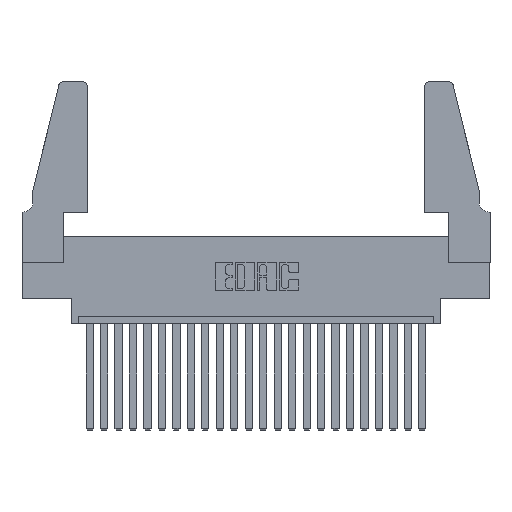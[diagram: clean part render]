
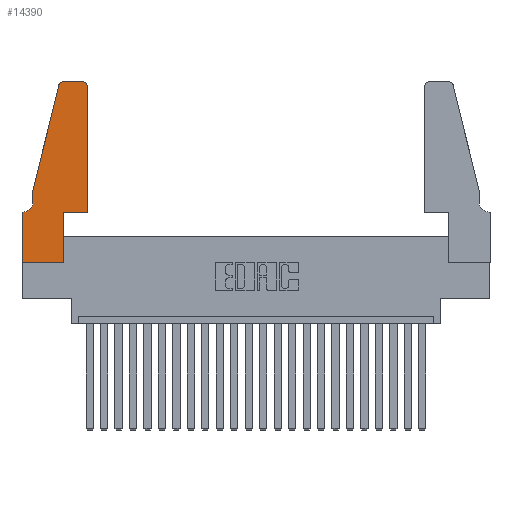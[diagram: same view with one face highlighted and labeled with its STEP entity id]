
A CAD part, top view. The second image highlights one B-rep face of the part: STEP entity #14390.
In plain terms, the highlighted planar face has unit normal (0, 0, 1).
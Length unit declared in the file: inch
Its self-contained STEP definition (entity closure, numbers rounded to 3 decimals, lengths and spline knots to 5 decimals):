
#561 = DIRECTION ( 'NONE',  ( 0., -1., 0. ) ) ;
#1116 = ORIENTED_EDGE ( 'NONE', *, *, #19696, .T. ) ;
#1305 = CARTESIAN_POINT ( 'NONE',  ( 0.4205, 1.22, 0.37 ) ) ;
#1450 = LINE ( 'NONE', #10555, #19457 ) ;
#1609 = VERTEX_POINT ( 'NONE', #7584 ) ;
#1665 = DIRECTION ( 'NONE',  ( 0., 0., 1. ) ) ;
#1676 = VERTEX_POINT ( 'NONE', #2249 ) ;
#1792 = EDGE_CURVE ( 'NONE', #5726, #1676, #8718, .T. ) ;
#1910 = DIRECTION ( 'NONE',  ( -0.239, -0.971, 0. ) ) ;
#2001 = CARTESIAN_POINT ( 'NONE',  ( 0., 0.35, 0.37 ) ) ;
#2024 = EDGE_LOOP ( 'NONE', ( #13230, #1116, #7763, #14770, #7213, #21778, #20930, #15979, #6445, #11899, #16811, #20175 ) ) ;
#2026 = EDGE_CURVE ( 'NONE', #1676, #17543, #18436, .T. ) ;
#2249 = CARTESIAN_POINT ( 'NONE',  ( 0., 0., 0.37 ) ) ;
#2500 = VECTOR ( 'NONE', #14699, 39.37008 ) ;
#3190 = VECTOR ( 'NONE', #20352, 39.37008 ) ;
#3226 = CARTESIAN_POINT ( 'NONE',  ( 0.284, 1.22, 0.37 ) ) ;
#3441 = CARTESIAN_POINT ( 'NONE',  ( 0., 0.35, 0.37 ) ) ;
#3914 = CIRCLE ( 'NONE', #15647, 0.03 ) ;
#4286 = EDGE_CURVE ( 'NONE', #7462, #20144, #18854, .T. ) ;
#4609 = EDGE_CURVE ( 'NONE', #1609, #6643, #7204, .T. ) ;
#4746 = VECTOR ( 'NONE', #1910, 39.37008 ) ;
#5726 = VERTEX_POINT ( 'NONE', #2001 ) ;
#6085 = DIRECTION ( 'NONE',  ( -1., 0., 0. ) ) ;
#6445 = ORIENTED_EDGE ( 'NONE', *, *, #7154, .T. ) ;
#6475 = CARTESIAN_POINT ( 'NONE',  ( 0., 0., 0.37 ) ) ;
#6643 = VERTEX_POINT ( 'NONE', #20934 ) ;
#7027 = DIRECTION ( 'NONE',  ( 0., 0., 1. ) ) ;
#7035 = LINE ( 'NONE', #17902, #19211 ) ;
#7154 = EDGE_CURVE ( 'NONE', #17543, #19338, #8972, .T. ) ;
#7204 = LINE ( 'NONE', #16432, #2500 ) ;
#7213 = ORIENTED_EDGE ( 'NONE', *, *, #11035, .T. ) ;
#7355 = CARTESIAN_POINT ( 'NONE',  ( 0.0755, 0.35, 0.37 ) ) ;
#7462 = VERTEX_POINT ( 'NONE', #18083 ) ;
#7584 = CARTESIAN_POINT ( 'NONE',  ( 0.4505, 0.35, 0.37 ) ) ;
#7623 = CARTESIAN_POINT ( 'NONE',  ( 0.0055, 0.35, 0.37 ) ) ;
#7763 = ORIENTED_EDGE ( 'NONE', *, *, #4286, .T. ) ;
#7776 = VERTEX_POINT ( 'NONE', #7623 ) ;
#8060 = DIRECTION ( 'NONE',  ( 1., 0., 0. ) ) ;
#8718 = LINE ( 'NONE', #9415, #11935 ) ;
#8972 = LINE ( 'NONE', #21272, #21488 ) ;
#9415 = CARTESIAN_POINT ( 'NONE',  ( 0., 0., 0.37 ) ) ;
#9448 = CARTESIAN_POINT ( 'NONE',  ( 0.2605, 1.25, 0.37 ) ) ;
#9596 = CIRCLE ( 'NONE', #12910, 0.03 ) ;
#9640 = VECTOR ( 'NONE', #15904, 39.37008 ) ;
#9907 = AXIS2_PLACEMENT_3D ( 'NONE', #22009, #16769, #18303 ) ;
#9958 = CARTESIAN_POINT ( 'NONE',  ( 0.2865, 0.35, 0.37 ) ) ;
#10555 = CARTESIAN_POINT ( 'NONE',  ( 0.0755, 0.5, 0.37 ) ) ;
#10727 = DIRECTION ( 'NONE',  ( 1., 0., 0. ) ) ;
#10754 = EDGE_CURVE ( 'NONE', #20144, #18884, #1450, .T. ) ;
#11035 = EDGE_CURVE ( 'NONE', #18884, #7776, #11817, .T. ) ;
#11658 = EDGE_CURVE ( 'NONE', #14169, #16993, #18050, .T. ) ;
#11817 = CIRCLE ( 'NONE', #9907, 0.07 ) ;
#11824 = DIRECTION ( 'NONE',  ( 1., 0., 0. ) ) ;
#11899 = ORIENTED_EDGE ( 'NONE', *, *, #15185, .T. ) ;
#11916 = DIRECTION ( 'NONE',  ( 1., 0., 0. ) ) ;
#11935 = VECTOR ( 'NONE', #18176, 39.37008 ) ;
#12910 = AXIS2_PLACEMENT_3D ( 'NONE', #3226, #1665, #11824 ) ;
#12967 = PLANE ( 'NONE',  #21171 ) ;
#13146 = VECTOR ( 'NONE', #6085, 39.37008 ) ;
#13230 = ORIENTED_EDGE ( 'NONE', *, *, #11658, .T. ) ;
#14169 = VERTEX_POINT ( 'NONE', #16796 ) ;
#14390 = ADVANCED_FACE ( 'NONE', ( #22054 ), #12967, .T. ) ;
#14699 = DIRECTION ( 'NONE',  ( 0., 1., 0. ) ) ;
#14770 = ORIENTED_EDGE ( 'NONE', *, *, #10754, .T. ) ;
#15185 = EDGE_CURVE ( 'NONE', #19338, #1609, #7035, .T. ) ;
#15647 = AXIS2_PLACEMENT_3D ( 'NONE', #1305, #7027, #11916 ) ;
#15904 = DIRECTION ( 'NONE',  ( -1., 0., 0. ) ) ;
#15979 = ORIENTED_EDGE ( 'NONE', *, *, #2026, .T. ) ;
#16432 = CARTESIAN_POINT ( 'NONE',  ( 0.4505, 0.35, 0.37 ) ) ;
#16769 = DIRECTION ( 'NONE',  ( 0., 0., -1. ) ) ;
#16796 = CARTESIAN_POINT ( 'NONE',  ( 0.4205, 1.25, 0.37 ) ) ;
#16811 = ORIENTED_EDGE ( 'NONE', *, *, #4609, .T. ) ;
#16993 = VERTEX_POINT ( 'NONE', #18685 ) ;
#17012 = EDGE_CURVE ( 'NONE', #6643, #14169, #3914, .T. ) ;
#17543 = VERTEX_POINT ( 'NONE', #20312 ) ;
#17678 = DIRECTION ( 'NONE',  ( 0., 1., 0. ) ) ;
#17902 = CARTESIAN_POINT ( 'NONE',  ( 0.4505, 0.35, 0.37 ) ) ;
#18050 = LINE ( 'NONE', #9448, #13146 ) ;
#18083 = CARTESIAN_POINT ( 'NONE',  ( 0.25487, 1.22718, 0.37 ) ) ;
#18176 = DIRECTION ( 'NONE',  ( 0., -1., 0. ) ) ;
#18303 = DIRECTION ( 'NONE',  ( -1., 0., 0. ) ) ;
#18436 = LINE ( 'NONE', #6475, #3190 ) ;
#18631 = CARTESIAN_POINT ( 'NONE',  ( 0.0755, 0.5, 0.37 ) ) ;
#18685 = CARTESIAN_POINT ( 'NONE',  ( 0.284, 1.25, 0.37 ) ) ;
#18854 = LINE ( 'NONE', #19200, #4746 ) ;
#18884 = VERTEX_POINT ( 'NONE', #21639 ) ;
#19017 = EDGE_CURVE ( 'NONE', #7776, #5726, #19081, .T. ) ;
#19081 = LINE ( 'NONE', #7355, #9640 ) ;
#19200 = CARTESIAN_POINT ( 'NONE',  ( 0.0755, 0.5, 0.37 ) ) ;
#19211 = VECTOR ( 'NONE', #8060, 39.37008 ) ;
#19338 = VERTEX_POINT ( 'NONE', #9958 ) ;
#19457 = VECTOR ( 'NONE', #561, 39.37008 ) ;
#19467 = DIRECTION ( 'NONE',  ( 0., 0., 1. ) ) ;
#19696 = EDGE_CURVE ( 'NONE', #16993, #7462, #9596, .T. ) ;
#20144 = VERTEX_POINT ( 'NONE', #18631 ) ;
#20175 = ORIENTED_EDGE ( 'NONE', *, *, #17012, .T. ) ;
#20312 = CARTESIAN_POINT ( 'NONE',  ( 0.2865, 0., 0.37 ) ) ;
#20352 = DIRECTION ( 'NONE',  ( 1., 0., 0. ) ) ;
#20930 = ORIENTED_EDGE ( 'NONE', *, *, #1792, .T. ) ;
#20934 = CARTESIAN_POINT ( 'NONE',  ( 0.4505, 1.22, 0.37 ) ) ;
#21171 = AXIS2_PLACEMENT_3D ( 'NONE', #3441, #19467, #10727 ) ;
#21272 = CARTESIAN_POINT ( 'NONE',  ( 0.2865, 0.35, 0.37 ) ) ;
#21488 = VECTOR ( 'NONE', #17678, 39.37008 ) ;
#21639 = CARTESIAN_POINT ( 'NONE',  ( 0.0755, 0.42, 0.37 ) ) ;
#21778 = ORIENTED_EDGE ( 'NONE', *, *, #19017, .T. ) ;
#22009 = CARTESIAN_POINT ( 'NONE',  ( 0.0055, 0.42, 0.37 ) ) ;
#22054 = FACE_OUTER_BOUND ( 'NONE', #2024, .T. ) ;
